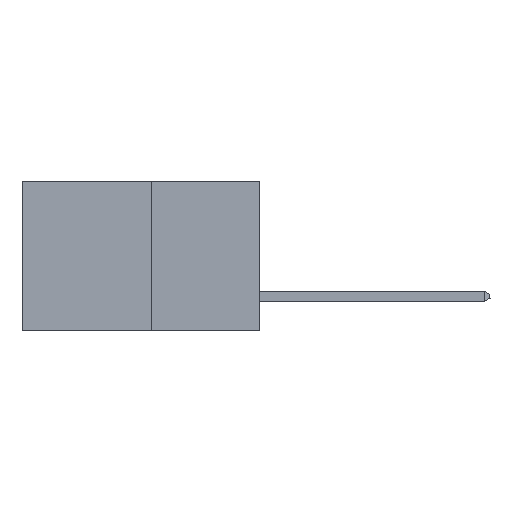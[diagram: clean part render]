
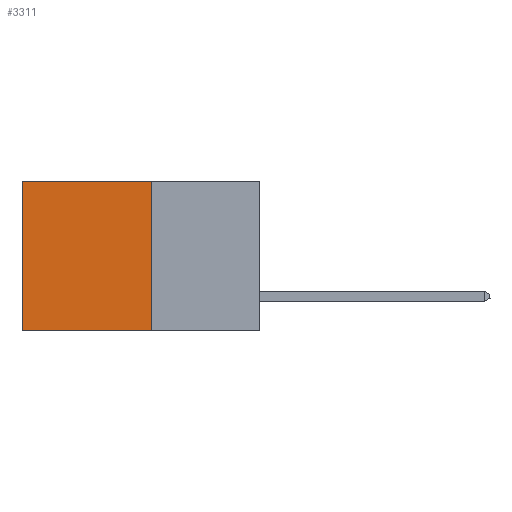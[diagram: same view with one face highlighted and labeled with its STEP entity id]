
A CAD part, left-side view. The second image highlights one B-rep face of the part: STEP entity #3311.
In plain terms, the highlighted planar face has unit normal (-1, 0, 0).
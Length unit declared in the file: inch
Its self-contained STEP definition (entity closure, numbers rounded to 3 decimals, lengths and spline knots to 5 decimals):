
#51 = VECTOR ( 'NONE', #28597, 39.37008 ) ;
#157 = VERTEX_POINT ( 'NONE', #13749 ) ;
#1970 = ORIENTED_EDGE ( 'NONE', *, *, #25174, .T. ) ;
#3311 = ADVANCED_FACE ( 'NONE', ( #7238 ), #4161, .F. ) ;
#3409 = DIRECTION ( 'NONE',  ( 0., 0., -1. ) ) ;
#3719 = ORIENTED_EDGE ( 'NONE', *, *, #27739, .T. ) ;
#3737 = EDGE_CURVE ( 'NONE', #16908, #157, #26233, .T. ) ;
#4161 = PLANE ( 'NONE',  #4760 ) ;
#4175 = CARTESIAN_POINT ( 'NONE',  ( 0.277, 0.27, 0. ) ) ;
#4760 = AXIS2_PLACEMENT_3D ( 'NONE', #20982, #18009, #30716 ) ;
#6595 = DIRECTION ( 'NONE',  ( 0., 1., 0. ) ) ;
#7164 = CARTESIAN_POINT ( 'NONE',  ( 0.277, 0.59, -0.37 ) ) ;
#7238 = FACE_OUTER_BOUND ( 'NONE', #25912, .T. ) ;
#8578 = ORIENTED_EDGE ( 'NONE', *, *, #16544, .F. ) ;
#11224 = VECTOR ( 'NONE', #3409, 39.37008 ) ;
#11539 = LINE ( 'NONE', #4175, #17903 ) ;
#11898 = CARTESIAN_POINT ( 'NONE',  ( 0.277, 0.27, -0.37 ) ) ;
#11906 = CARTESIAN_POINT ( 'NONE',  ( 0.277, 0.27, -0.37 ) ) ;
#12156 = VERTEX_POINT ( 'NONE', #20861 ) ;
#13223 = DIRECTION ( 'NONE',  ( 0., 1., 0. ) ) ;
#13749 = CARTESIAN_POINT ( 'NONE',  ( 0.277, 0.59, -0.37 ) ) ;
#15890 = ORIENTED_EDGE ( 'NONE', *, *, #3737, .F. ) ;
#16544 = EDGE_CURVE ( 'NONE', #27941, #16908, #23926, .T. ) ;
#16908 = VERTEX_POINT ( 'NONE', #11906 ) ;
#17903 = VECTOR ( 'NONE', #6595, 39.37008 ) ;
#18009 = DIRECTION ( 'NONE',  ( 1., 0., 0. ) ) ;
#19149 = LINE ( 'NONE', #7164, #51 ) ;
#19918 = VECTOR ( 'NONE', #13223, 39.37008 ) ;
#20161 = CARTESIAN_POINT ( 'NONE',  ( 0.277, 0.27, -0.37 ) ) ;
#20861 = CARTESIAN_POINT ( 'NONE',  ( 0.277, 0.59, 0. ) ) ;
#20982 = CARTESIAN_POINT ( 'NONE',  ( 0.277, 0.27, -0.37 ) ) ;
#21639 = CARTESIAN_POINT ( 'NONE',  ( 0.277, 0.27, 0. ) ) ;
#23926 = LINE ( 'NONE', #20161, #11224 ) ;
#25174 = EDGE_CURVE ( 'NONE', #12156, #157, #19149, .T. ) ;
#25912 = EDGE_LOOP ( 'NONE', ( #1970, #15890, #8578, #3719 ) ) ;
#26233 = LINE ( 'NONE', #11898, #19918 ) ;
#27739 = EDGE_CURVE ( 'NONE', #27941, #12156, #11539, .T. ) ;
#27941 = VERTEX_POINT ( 'NONE', #21639 ) ;
#28597 = DIRECTION ( 'NONE',  ( 0., 0., -1. ) ) ;
#30716 = DIRECTION ( 'NONE',  ( 0., 0., -1. ) ) ;
